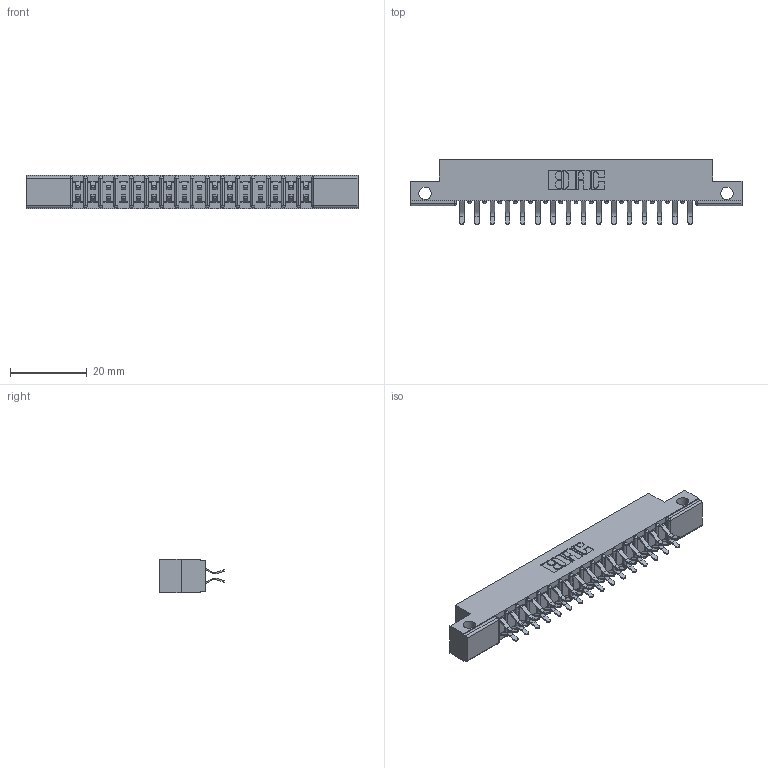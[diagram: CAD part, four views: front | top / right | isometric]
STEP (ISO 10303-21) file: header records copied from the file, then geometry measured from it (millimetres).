
FILE_DESCRIPTION (( 'STEP AP203' ), '1' );
FILE_NAME ('357-032-456-212.STEP', '2020-10-03T15:05:35', ( '' ), ( '' ), 'SwSTEP 2.0', 'SolidWorks 2020', '' );
FILE_SCHEMA (( 'CONFIG_CONTROL_DESIGN' ));
Length unit declared in the file: inch
Products named in the file (3): 307-290-001_556; 357-032-456-212; 307 Part_.128 Dia Side Mounting Holes
Assembly tree (33 placements, depth 2):
  357-032-456-212
    307 Part_.128 Dia Side Mounting Holes
    307-290-001_556  x32
Bounding box: 86.41 x 16.97 x 8.71 mm (x, y, z)
Volume: 5571.2 mm3; surface area: 9356.9 mm2
Topology: 33 solids, 33 shells, 1735 faces, 4867 edges, 3154 vertices
Faces by surface type: plane 1126, cylinder 575, sphere 34
Entity records: 17540 total; most frequent: CARTESIAN_POINT 2876, ORIENTED_EDGE 2846, DIRECTION 2829, EDGE_CURVE 1423, LINE 1079, VECTOR 1079, VERTEX_POINT 922, AXIS2_PLACEMENT_3D 875
